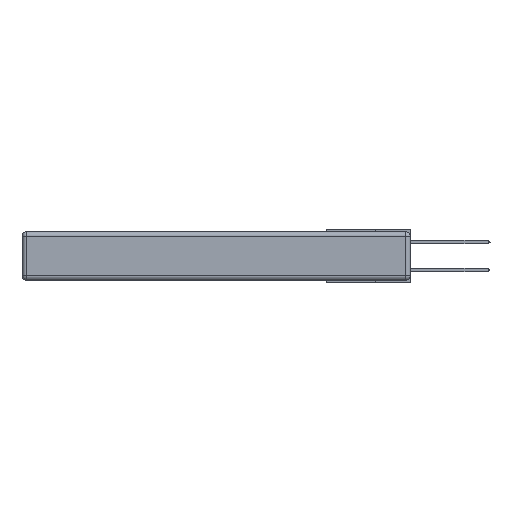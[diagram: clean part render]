
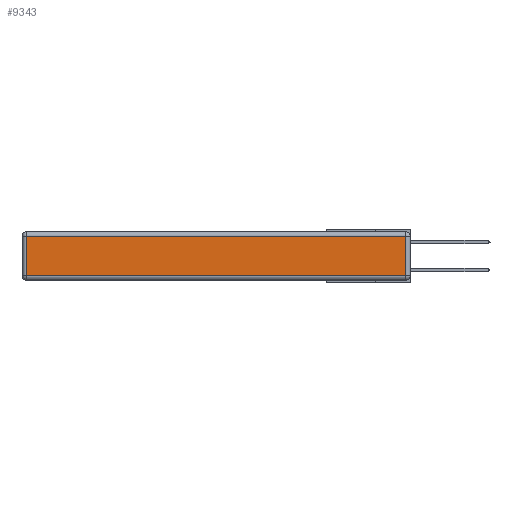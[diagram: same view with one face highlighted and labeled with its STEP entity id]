
A CAD part, left-side view. The second image highlights one B-rep face of the part: STEP entity #9343.
In plain terms, the highlighted planar face has unit normal (-1, 0, 0).
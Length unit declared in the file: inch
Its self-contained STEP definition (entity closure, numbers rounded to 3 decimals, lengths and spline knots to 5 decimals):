
#77 = DIRECTION ( 'NONE',  ( -1., 0., 0. ) ) ;
#258 = LINE ( 'NONE', #2950, #19703 ) ;
#445 = VECTOR ( 'NONE', #17937, 39.37008 ) ;
#1344 = LINE ( 'NONE', #1494, #18355 ) ;
#1494 = CARTESIAN_POINT ( 'NONE',  ( 0., 0., -0.313 ) ) ;
#1689 = CARTESIAN_POINT ( 'NONE',  ( 0., 0., -0.343 ) ) ;
#2422 = CARTESIAN_POINT ( 'NONE',  ( 0., 2.72, -0.03 ) ) ;
#2765 = CARTESIAN_POINT ( 'NONE',  ( 0., 0.03, -0.343 ) ) ;
#2950 = CARTESIAN_POINT ( 'NONE',  ( 0., 2.75, -0.03 ) ) ;
#6558 = CARTESIAN_POINT ( 'NONE',  ( 0., 2.72, -0.313 ) ) ;
#8869 = ORIENTED_EDGE ( 'NONE', *, *, #9797, .T. ) ;
#9174 = CARTESIAN_POINT ( 'NONE',  ( 0., 2.72, -0.343 ) ) ;
#9343 = ADVANCED_FACE ( 'NONE', ( #21970 ), #32552, .T. ) ;
#9397 = DIRECTION ( 'NONE',  ( 0., 0., -1. ) ) ;
#9797 = EDGE_CURVE ( 'NONE', #28903, #20707, #32740, .T. ) ;
#11617 = VECTOR ( 'NONE', #9397, 39.37008 ) ;
#12007 = DIRECTION ( 'NONE',  ( 0., -1., 0. ) ) ;
#12327 = EDGE_CURVE ( 'NONE', #27364, #31988, #29367, .T. ) ;
#17937 = DIRECTION ( 'NONE',  ( 0., 0., 1. ) ) ;
#18355 = VECTOR ( 'NONE', #12007, 39.37008 ) ;
#19242 = AXIS2_PLACEMENT_3D ( 'NONE', #1689, #77, #30882 ) ;
#19703 = VECTOR ( 'NONE', #23494, 39.37008 ) ;
#20707 = VERTEX_POINT ( 'NONE', #22464 ) ;
#21355 = EDGE_CURVE ( 'NONE', #20707, #27364, #258, .T. ) ;
#21970 = FACE_OUTER_BOUND ( 'NONE', #32938, .T. ) ;
#22464 = CARTESIAN_POINT ( 'NONE',  ( 0., 0.03, -0.03 ) ) ;
#23494 = DIRECTION ( 'NONE',  ( 0., 1., 0. ) ) ;
#24192 = EDGE_CURVE ( 'NONE', #31988, #28903, #1344, .T. ) ;
#27364 = VERTEX_POINT ( 'NONE', #2422 ) ;
#28207 = ORIENTED_EDGE ( 'NONE', *, *, #24192, .T. ) ;
#28903 = VERTEX_POINT ( 'NONE', #30178 ) ;
#29367 = LINE ( 'NONE', #9174, #11617 ) ;
#30178 = CARTESIAN_POINT ( 'NONE',  ( 0., 0.03, -0.313 ) ) ;
#30882 = DIRECTION ( 'NONE',  ( 0., 0., 1. ) ) ;
#31988 = VERTEX_POINT ( 'NONE', #6558 ) ;
#32552 = PLANE ( 'NONE',  #19242 ) ;
#32740 = LINE ( 'NONE', #2765, #445 ) ;
#32938 = EDGE_LOOP ( 'NONE', ( #28207, #8869, #33412, #33304 ) ) ;
#33304 = ORIENTED_EDGE ( 'NONE', *, *, #12327, .T. ) ;
#33412 = ORIENTED_EDGE ( 'NONE', *, *, #21355, .T. ) ;
